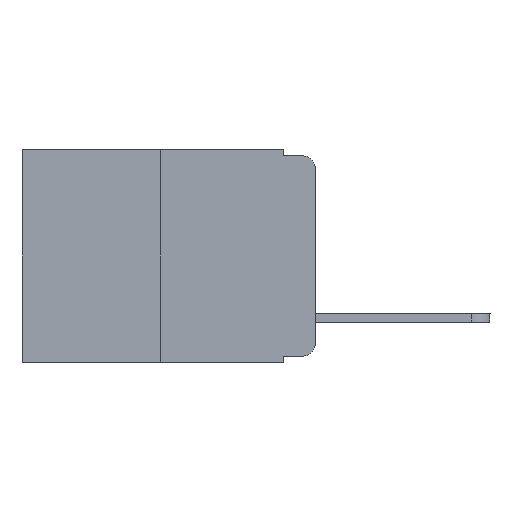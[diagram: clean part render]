
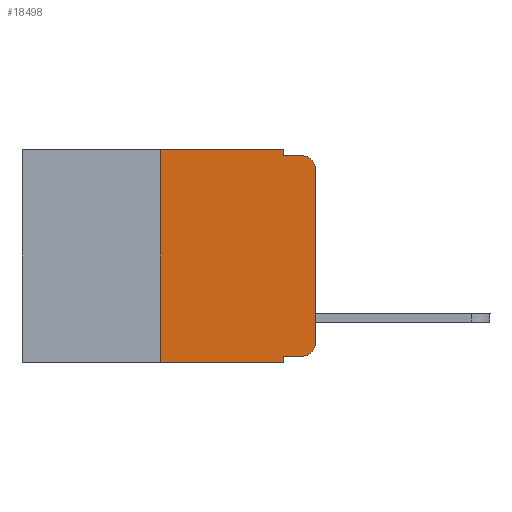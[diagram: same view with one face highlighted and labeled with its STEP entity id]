
A CAD part, left-side view. The second image highlights one B-rep face of the part: STEP entity #18498.
In plain terms, the highlighted planar face has unit normal (-1, 0, 0).
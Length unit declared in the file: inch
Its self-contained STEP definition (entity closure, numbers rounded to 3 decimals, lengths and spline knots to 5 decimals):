
#44 = DIRECTION ( 'NONE',  ( -1., 0., 0. ) ) ;
#68 = CARTESIAN_POINT ( 'NONE',  ( 0., 0.051, -0.333 ) ) ;
#595 = EDGE_CURVE ( 'NONE', #5585, #20422, #3058, .T. ) ;
#691 = EDGE_CURVE ( 'NONE', #15126, #7755, #19006, .T. ) ;
#829 = VERTEX_POINT ( 'NONE', #5636 ) ;
#912 = VERTEX_POINT ( 'NONE', #10935 ) ;
#928 = VERTEX_POINT ( 'NONE', #21268 ) ;
#1038 = CARTESIAN_POINT ( 'NONE',  ( 0., 0.02, -0.333 ) ) ;
#1597 = CARTESIAN_POINT ( 'NONE',  ( 0., 0.02, -0.03 ) ) ;
#1712 = VECTOR ( 'NONE', #21434, 39.37008 ) ;
#2111 = VERTEX_POINT ( 'NONE', #20796 ) ;
#2311 = CARTESIAN_POINT ( 'NONE',  ( 0., 0.02, -0.313 ) ) ;
#2383 = DIRECTION ( 'NONE',  ( 0., 0., -1. ) ) ;
#2744 = EDGE_LOOP ( 'NONE', ( #11573, #8252, #5290, #7448, #3370, #20654, #6521, #12562, #18180, #12507 ) ) ;
#2746 = PLANE ( 'NONE',  #4136 ) ;
#2815 = DIRECTION ( 'NONE',  ( 0., 0., -1. ) ) ;
#3058 = LINE ( 'NONE', #21360, #1712 ) ;
#3370 = ORIENTED_EDGE ( 'NONE', *, *, #21068, .F. ) ;
#3846 = CIRCLE ( 'NONE', #13511, 0.02 ) ;
#3962 = CARTESIAN_POINT ( 'NONE',  ( 0., 0.25, -0.343 ) ) ;
#4136 = AXIS2_PLACEMENT_3D ( 'NONE', #19498, #4484, #2815 ) ;
#4168 = DIRECTION ( 'NONE',  ( 0., -1., 0. ) ) ;
#4271 = CARTESIAN_POINT ( 'NONE',  ( 0., 0.051, -0.01 ) ) ;
#4484 = DIRECTION ( 'NONE',  ( 1., 0., 0. ) ) ;
#4726 = CARTESIAN_POINT ( 'NONE',  ( 0., 0.051, -0.333 ) ) ;
#4913 = LINE ( 'NONE', #19708, #12524 ) ;
#4968 = DIRECTION ( 'NONE',  ( 0., 0., -1. ) ) ;
#5049 = AXIS2_PLACEMENT_3D ( 'NONE', #1597, #44, #4968 ) ;
#5290 = ORIENTED_EDGE ( 'NONE', *, *, #18232, .F. ) ;
#5391 = CARTESIAN_POINT ( 'NONE',  ( 0., 0.051, -0.01 ) ) ;
#5467 = CARTESIAN_POINT ( 'NONE',  ( 0., 0.051, 0. ) ) ;
#5585 = VERTEX_POINT ( 'NONE', #3962 ) ;
#5636 = CARTESIAN_POINT ( 'NONE',  ( 0., 0., -0.03 ) ) ;
#5849 = LINE ( 'NONE', #7440, #6129 ) ;
#6129 = VECTOR ( 'NONE', #12654, 39.37008 ) ;
#6521 = ORIENTED_EDGE ( 'NONE', *, *, #595, .T. ) ;
#6738 = VECTOR ( 'NONE', #4168, 39.37008 ) ;
#6913 = EDGE_CURVE ( 'NONE', #15126, #20422, #9626, .T. ) ;
#7102 = CARTESIAN_POINT ( 'NONE',  ( 0., 0.051, 0. ) ) ;
#7142 = DIRECTION ( 'NONE',  ( 0., 0., -1. ) ) ;
#7440 = CARTESIAN_POINT ( 'NONE',  ( 0., 0.051, 0. ) ) ;
#7448 = ORIENTED_EDGE ( 'NONE', *, *, #9267, .F. ) ;
#7601 = EDGE_CURVE ( 'NONE', #7755, #912, #3846, .T. ) ;
#7714 = DIRECTION ( 'NONE',  ( 0., -1., 0. ) ) ;
#7755 = VERTEX_POINT ( 'NONE', #1038 ) ;
#7861 = VECTOR ( 'NONE', #7714, 39.37008 ) ;
#8023 = VERTEX_POINT ( 'NONE', #5391 ) ;
#8252 = ORIENTED_EDGE ( 'NONE', *, *, #14650, .T. ) ;
#9151 = DIRECTION ( 'NONE',  ( 0., 0., 1. ) ) ;
#9267 = EDGE_CURVE ( 'NONE', #11665, #8023, #5849, .T. ) ;
#9601 = VECTOR ( 'NONE', #17154, 39.37008 ) ;
#9626 = LINE ( 'NONE', #5467, #17724 ) ;
#9695 = DIRECTION ( 'NONE',  ( 0., 0., 1. ) ) ;
#10935 = CARTESIAN_POINT ( 'NONE',  ( 0., 0., -0.313 ) ) ;
#11573 = ORIENTED_EDGE ( 'NONE', *, *, #20612, .T. ) ;
#11665 = VERTEX_POINT ( 'NONE', #7102 ) ;
#12058 = CARTESIAN_POINT ( 'NONE',  ( 0., 0.25, 0. ) ) ;
#12504 = LINE ( 'NONE', #19465, #6738 ) ;
#12507 = ORIENTED_EDGE ( 'NONE', *, *, #7601, .T. ) ;
#12524 = VECTOR ( 'NONE', #9695, 39.37008 ) ;
#12562 = ORIENTED_EDGE ( 'NONE', *, *, #6913, .F. ) ;
#12604 = VECTOR ( 'NONE', #9151, 39.37008 ) ;
#12654 = DIRECTION ( 'NONE',  ( 0., 0., -1. ) ) ;
#13511 = AXIS2_PLACEMENT_3D ( 'NONE', #2311, #17543, #2383 ) ;
#14650 = EDGE_CURVE ( 'NONE', #829, #928, #18496, .T. ) ;
#15126 = VERTEX_POINT ( 'NONE', #4726 ) ;
#17025 = FACE_OUTER_BOUND ( 'NONE', #2744, .T. ) ;
#17154 = DIRECTION ( 'NONE',  ( 0., -1., 0. ) ) ;
#17543 = DIRECTION ( 'NONE',  ( -1., 0., 0. ) ) ;
#17632 = EDGE_CURVE ( 'NONE', #5585, #2111, #19408, .T. ) ;
#17724 = VECTOR ( 'NONE', #7142, 39.37008 ) ;
#17739 = CARTESIAN_POINT ( 'NONE',  ( 0., 0.051, -0.343 ) ) ;
#18180 = ORIENTED_EDGE ( 'NONE', *, *, #691, .T. ) ;
#18232 = EDGE_CURVE ( 'NONE', #8023, #928, #19363, .T. ) ;
#18496 = CIRCLE ( 'NONE', #5049, 0.02 ) ;
#18498 = ADVANCED_FACE ( 'NONE', ( #17025 ), #2746, .F. ) ;
#19006 = LINE ( 'NONE', #68, #9601 ) ;
#19363 = LINE ( 'NONE', #4271, #7861 ) ;
#19408 = LINE ( 'NONE', #12058, #12604 ) ;
#19465 = CARTESIAN_POINT ( 'NONE',  ( 0., 0.473, 0. ) ) ;
#19498 = CARTESIAN_POINT ( 'NONE',  ( 0., 0.473, 0. ) ) ;
#19708 = CARTESIAN_POINT ( 'NONE',  ( 0., 0., 0. ) ) ;
#20422 = VERTEX_POINT ( 'NONE', #17739 ) ;
#20612 = EDGE_CURVE ( 'NONE', #912, #829, #4913, .T. ) ;
#20654 = ORIENTED_EDGE ( 'NONE', *, *, #17632, .F. ) ;
#20796 = CARTESIAN_POINT ( 'NONE',  ( 0., 0.25, 0. ) ) ;
#21068 = EDGE_CURVE ( 'NONE', #2111, #11665, #12504, .T. ) ;
#21268 = CARTESIAN_POINT ( 'NONE',  ( 0., 0.02, -0.01 ) ) ;
#21360 = CARTESIAN_POINT ( 'NONE',  ( 0., 0.473, -0.343 ) ) ;
#21434 = DIRECTION ( 'NONE',  ( 0., -1., 0. ) ) ;
